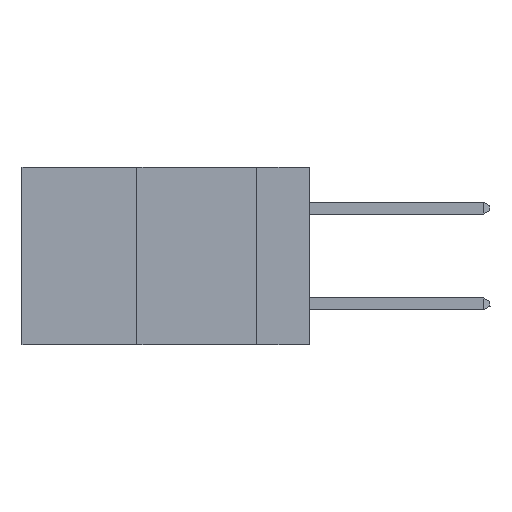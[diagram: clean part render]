
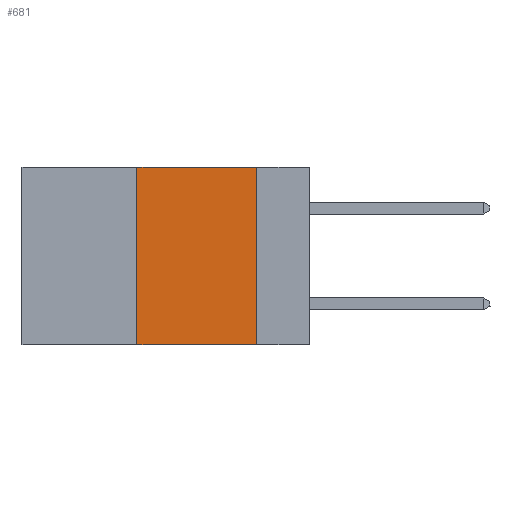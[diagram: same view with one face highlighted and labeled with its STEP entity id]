
A CAD part, left-side view. The second image highlights one B-rep face of the part: STEP entity #681.
In plain terms, the highlighted planar face has unit normal (-1, 0, 0).
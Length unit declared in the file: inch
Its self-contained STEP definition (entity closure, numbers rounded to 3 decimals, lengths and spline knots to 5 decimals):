
#420 = DIRECTION ( 'NONE',  ( 0., 0., -1. ) ) ;
#581 = VECTOR ( 'NONE', #2072, 39.37008 ) ;
#681 = ADVANCED_FACE ( 'NONE', ( #7393 ), #7848, .F. ) ;
#692 = ORIENTED_EDGE ( 'NONE', *, *, #5725, .F. ) ;
#868 = CARTESIAN_POINT ( 'NONE',  ( 0., 0.36, -0.37 ) ) ;
#869 = ORIENTED_EDGE ( 'NONE', *, *, #5524, .F. ) ;
#987 = ORIENTED_EDGE ( 'NONE', *, *, #5249, .F. ) ;
#1009 = ORIENTED_EDGE ( 'NONE', *, *, #4718, .T. ) ;
#2072 = DIRECTION ( 'NONE',  ( 0., 0., -1. ) ) ;
#2347 = CARTESIAN_POINT ( 'NONE',  ( 0., 0.6, -0.37 ) ) ;
#2382 = LINE ( 'NONE', #2616, #7746 ) ;
#2429 = VERTEX_POINT ( 'NONE', #868 ) ;
#2557 = CARTESIAN_POINT ( 'NONE',  ( 0., 0.11, 0. ) ) ;
#2581 = DIRECTION ( 'NONE',  ( 0., 0., 1. ) ) ;
#2616 = CARTESIAN_POINT ( 'NONE',  ( 0., 0.36, 0. ) ) ;
#2806 = EDGE_LOOP ( 'NONE', ( #692, #987, #869, #1009 ) ) ;
#3580 = VECTOR ( 'NONE', #7704, 39.37008 ) ;
#4209 = LINE ( 'NONE', #2557, #581 ) ;
#4594 = DIRECTION ( 'NONE',  ( 1., 0., 0. ) ) ;
#4718 = EDGE_CURVE ( 'NONE', #2429, #4720, #5408, .T. ) ;
#4720 = VERTEX_POINT ( 'NONE', #8665 ) ;
#4745 = CARTESIAN_POINT ( 'NONE',  ( 0., 0.6, 0. ) ) ;
#4840 = VERTEX_POINT ( 'NONE', #7259 ) ;
#4958 = LINE ( 'NONE', #7919, #8283 ) ;
#5067 = VERTEX_POINT ( 'NONE', #7596 ) ;
#5249 = EDGE_CURVE ( 'NONE', #5067, #4840, #4958, .T. ) ;
#5408 = LINE ( 'NONE', #2347, #3580 ) ;
#5524 = EDGE_CURVE ( 'NONE', #2429, #5067, #2382, .T. ) ;
#5707 = AXIS2_PLACEMENT_3D ( 'NONE', #4745, #4594, #420 ) ;
#5725 = EDGE_CURVE ( 'NONE', #4840, #4720, #4209, .T. ) ;
#6530 = DIRECTION ( 'NONE',  ( 0., -1., 0. ) ) ;
#7259 = CARTESIAN_POINT ( 'NONE',  ( 0., 0.11, 0. ) ) ;
#7393 = FACE_OUTER_BOUND ( 'NONE', #2806, .T. ) ;
#7596 = CARTESIAN_POINT ( 'NONE',  ( 0., 0.36, 0. ) ) ;
#7704 = DIRECTION ( 'NONE',  ( 0., -1., 0. ) ) ;
#7746 = VECTOR ( 'NONE', #2581, 39.37008 ) ;
#7848 = PLANE ( 'NONE',  #5707 ) ;
#7919 = CARTESIAN_POINT ( 'NONE',  ( 0., 0.6, 0. ) ) ;
#8283 = VECTOR ( 'NONE', #6530, 39.37008 ) ;
#8665 = CARTESIAN_POINT ( 'NONE',  ( 0., 0.11, -0.37 ) ) ;
